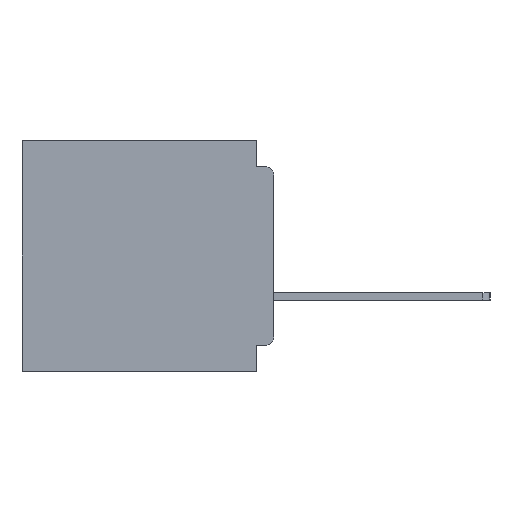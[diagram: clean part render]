
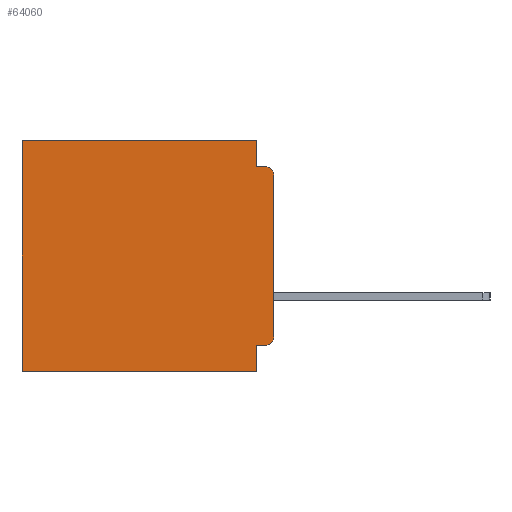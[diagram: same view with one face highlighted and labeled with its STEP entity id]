
A CAD part, left-side view. The second image highlights one B-rep face of the part: STEP entity #64060.
In plain terms, the highlighted planar face has unit normal (-1, 0, 0).
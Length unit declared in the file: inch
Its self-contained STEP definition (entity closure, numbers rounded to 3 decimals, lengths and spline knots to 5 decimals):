
#513 = VECTOR ( 'NONE', #58928, 39.37008 ) ;
#885 = DIRECTION ( 'NONE',  ( -1., 0., 0. ) ) ;
#2148 = VERTEX_POINT ( 'NONE', #63410 ) ;
#2239 = CARTESIAN_POINT ( 'NONE',  ( 0.3, 0., -0.045 ) ) ;
#2956 = DIRECTION ( 'NONE',  ( 0., 0., -1. ) ) ;
#3287 = VERTEX_POINT ( 'NONE', #44093 ) ;
#4339 = CIRCLE ( 'NONE', #6913, 0.015 ) ;
#4617 = DIRECTION ( 'NONE',  ( 0., 0., -1. ) ) ;
#5178 = DIRECTION ( 'NONE',  ( 0., 0., -1. ) ) ;
#6218 = EDGE_CURVE ( 'NONE', #3287, #47604, #11767, .T. ) ;
#6318 = EDGE_CURVE ( 'NONE', #12140, #22753, #46533, .T. ) ;
#6913 = AXIS2_PLACEMENT_3D ( 'NONE', #31853, #885, #37029 ) ;
#7645 = CARTESIAN_POINT ( 'NONE',  ( 0.3, 0., -0.355 ) ) ;
#7795 = PLANE ( 'NONE',  #60153 ) ;
#11767 = LINE ( 'NONE', #51583, #65038 ) ;
#12084 = DIRECTION ( 'NONE',  ( 0., 1., 0. ) ) ;
#12140 = VERTEX_POINT ( 'NONE', #45988 ) ;
#12297 = DIRECTION ( 'NONE',  ( 0., 0., -1. ) ) ;
#12984 = CARTESIAN_POINT ( 'NONE',  ( 0.3, 0., -0.4 ) ) ;
#13580 = LINE ( 'NONE', #7645, #66896 ) ;
#13701 = DIRECTION ( 'NONE',  ( 0., 0., -1. ) ) ;
#15512 = VECTOR ( 'NONE', #13701, 39.37008 ) ;
#16054 = LINE ( 'NONE', #61501, #19295 ) ;
#17152 = LINE ( 'NONE', #49835, #15512 ) ;
#18193 = DIRECTION ( 'NONE',  ( 1., 0., 0. ) ) ;
#18362 = VERTEX_POINT ( 'NONE', #29141 ) ;
#19295 = VECTOR ( 'NONE', #4617, 39.37008 ) ;
#20563 = CARTESIAN_POINT ( 'NONE',  ( 0.3, 0.031, 0. ) ) ;
#20661 = EDGE_CURVE ( 'NONE', #18362, #38737, #13580, .T. ) ;
#20680 = DIRECTION ( 'NONE',  ( 0., 1., 0. ) ) ;
#22258 = CARTESIAN_POINT ( 'NONE',  ( 0.3, 0., 0. ) ) ;
#22668 = ORIENTED_EDGE ( 'NONE', *, *, #42136, .F. ) ;
#22753 = VERTEX_POINT ( 'NONE', #43818 ) ;
#23016 = CARTESIAN_POINT ( 'NONE',  ( 0.3, 0.031, -0.355 ) ) ;
#24037 = VERTEX_POINT ( 'NONE', #34148 ) ;
#24821 = VERTEX_POINT ( 'NONE', #61550 ) ;
#24962 = ORIENTED_EDGE ( 'NONE', *, *, #55474, .F. ) ;
#25502 = ORIENTED_EDGE ( 'NONE', *, *, #57180, .T. ) ;
#29141 = CARTESIAN_POINT ( 'NONE',  ( 0.3, 0.015, -0.355 ) ) ;
#29380 = VERTEX_POINT ( 'NONE', #53031 ) ;
#30562 = VECTOR ( 'NONE', #12297, 39.37008 ) ;
#30651 = FACE_OUTER_BOUND ( 'NONE', #52939, .T. ) ;
#31853 = CARTESIAN_POINT ( 'NONE',  ( 0.3, 0.015, -0.34 ) ) ;
#32345 = ORIENTED_EDGE ( 'NONE', *, *, #40733, .T. ) ;
#32514 = EDGE_CURVE ( 'NONE', #24037, #29380, #16054, .T. ) ;
#33686 = CARTESIAN_POINT ( 'NONE',  ( 0.3, 0.437, -0.4 ) ) ;
#33932 = DIRECTION ( 'NONE',  ( -1., 0., 0. ) ) ;
#34148 = CARTESIAN_POINT ( 'NONE',  ( 0.3, 0., -0.06 ) ) ;
#37029 = DIRECTION ( 'NONE',  ( 0., 0., -1. ) ) ;
#38024 = CARTESIAN_POINT ( 'NONE',  ( 0.3, 0.031, -0.4 ) ) ;
#38097 = ORIENTED_EDGE ( 'NONE', *, *, #32514, .F. ) ;
#38737 = VERTEX_POINT ( 'NONE', #23016 ) ;
#38847 = LINE ( 'NONE', #20563, #64668 ) ;
#40733 = EDGE_CURVE ( 'NONE', #22753, #47604, #17152, .T. ) ;
#41767 = LINE ( 'NONE', #2239, #513 ) ;
#42136 = EDGE_CURVE ( 'NONE', #12140, #2148, #38847, .T. ) ;
#43818 = CARTESIAN_POINT ( 'NONE',  ( 0.3, 0.437, 0. ) ) ;
#44093 = CARTESIAN_POINT ( 'NONE',  ( 0.3, 0.031, -0.4 ) ) ;
#45988 = CARTESIAN_POINT ( 'NONE',  ( 0.3, 0.031, 0. ) ) ;
#46533 = LINE ( 'NONE', #22258, #58593 ) ;
#47604 = VERTEX_POINT ( 'NONE', #33686 ) ;
#49287 = ORIENTED_EDGE ( 'NONE', *, *, #57580, .T. ) ;
#49835 = CARTESIAN_POINT ( 'NONE',  ( 0.3, 0.437, -0.4 ) ) ;
#49963 = ORIENTED_EDGE ( 'NONE', *, *, #6318, .T. ) ;
#51583 = CARTESIAN_POINT ( 'NONE',  ( 0.3, 0., -0.4 ) ) ;
#51662 = ORIENTED_EDGE ( 'NONE', *, *, #20661, .F. ) ;
#52632 = ORIENTED_EDGE ( 'NONE', *, *, #6218, .F. ) ;
#52901 = CIRCLE ( 'NONE', #61378, 0.015 ) ;
#52939 = EDGE_LOOP ( 'NONE', ( #38097, #25502, #53563, #22668, #49963, #32345, #52632, #24962, #51662, #49287 ) ) ;
#53031 = CARTESIAN_POINT ( 'NONE',  ( 0.3, 0., -0.34 ) ) ;
#53563 = ORIENTED_EDGE ( 'NONE', *, *, #56127, .F. ) ;
#54317 = DIRECTION ( 'NONE',  ( 0., 0., -1. ) ) ;
#55474 = EDGE_CURVE ( 'NONE', #38737, #3287, #56409, .T. ) ;
#56127 = EDGE_CURVE ( 'NONE', #2148, #24821, #41767, .T. ) ;
#56409 = LINE ( 'NONE', #38024, #30562 ) ;
#57180 = EDGE_CURVE ( 'NONE', #24037, #24821, #52901, .T. ) ;
#57580 = EDGE_CURVE ( 'NONE', #18362, #29380, #4339, .T. ) ;
#58593 = VECTOR ( 'NONE', #12084, 39.37008 ) ;
#58928 = DIRECTION ( 'NONE',  ( 0., -1., 0. ) ) ;
#60153 = AXIS2_PLACEMENT_3D ( 'NONE', #12984, #18193, #54317 ) ;
#61378 = AXIS2_PLACEMENT_3D ( 'NONE', #64816, #33932, #2956 ) ;
#61501 = CARTESIAN_POINT ( 'NONE',  ( 0.3, 0., -0.4 ) ) ;
#61550 = CARTESIAN_POINT ( 'NONE',  ( 0.3, 0.015, -0.045 ) ) ;
#63410 = CARTESIAN_POINT ( 'NONE',  ( 0.3, 0.031, -0.045 ) ) ;
#64060 = ADVANCED_FACE ( 'NONE', ( #30651 ), #7795, .F. ) ;
#64513 = DIRECTION ( 'NONE',  ( 0., 1., 0. ) ) ;
#64668 = VECTOR ( 'NONE', #5178, 39.37008 ) ;
#64816 = CARTESIAN_POINT ( 'NONE',  ( 0.3, 0.015, -0.06 ) ) ;
#65038 = VECTOR ( 'NONE', #20680, 39.37008 ) ;
#66896 = VECTOR ( 'NONE', #64513, 39.37008 ) ;
